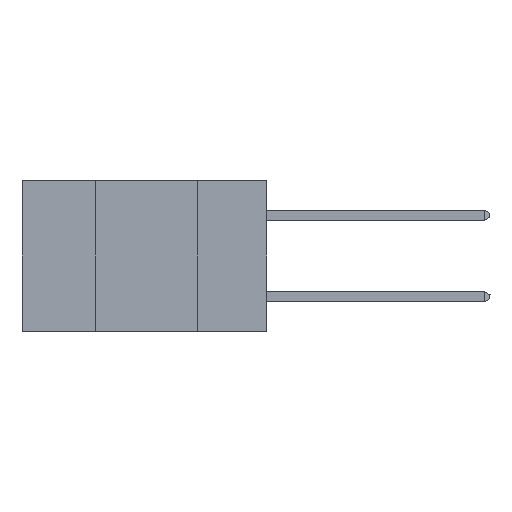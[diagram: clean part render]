
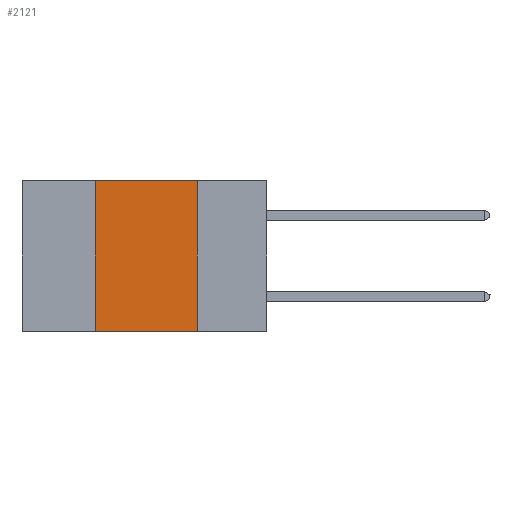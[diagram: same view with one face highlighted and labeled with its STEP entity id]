
A CAD part, left-side view. The second image highlights one B-rep face of the part: STEP entity #2121.
In plain terms, the highlighted planar face has unit normal (-1, 0, 0).
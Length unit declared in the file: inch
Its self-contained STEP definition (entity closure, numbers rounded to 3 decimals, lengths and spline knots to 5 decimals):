
#1467 = LINE ( 'NONE', #8343, #33028 ) ;
#2121 = ADVANCED_FACE ( 'NONE', ( #2876 ), #19632, .F. ) ;
#2876 = FACE_OUTER_BOUND ( 'NONE', #6727, .T. ) ;
#3193 = VECTOR ( 'NONE', #22017, 39.37008 ) ;
#6084 = LINE ( 'NONE', #10353, #6583 ) ;
#6583 = VECTOR ( 'NONE', #26523, 39.37008 ) ;
#6727 = EDGE_LOOP ( 'NONE', ( #13665, #14573, #33638, #40450 ) ) ;
#7032 = EDGE_CURVE ( 'NONE', #20802, #23685, #1467, .T. ) ;
#8343 = CARTESIAN_POINT ( 'NONE',  ( 0., 0.6, 0. ) ) ;
#10353 = CARTESIAN_POINT ( 'NONE',  ( 0., 0.42, 0. ) ) ;
#10369 = DIRECTION ( 'NONE',  ( 1., 0., 0. ) ) ;
#13665 = ORIENTED_EDGE ( 'NONE', *, *, #32735, .F. ) ;
#14012 = VERTEX_POINT ( 'NONE', #22303 ) ;
#14573 = ORIENTED_EDGE ( 'NONE', *, *, #7032, .F. ) ;
#19632 = PLANE ( 'NONE',  #36385 ) ;
#20323 = CARTESIAN_POINT ( 'NONE',  ( 0., 0.6, 0. ) ) ;
#20802 = VERTEX_POINT ( 'NONE', #41307 ) ;
#22017 = DIRECTION ( 'NONE',  ( 0., 0., -1. ) ) ;
#22303 = CARTESIAN_POINT ( 'NONE',  ( 0., 0.17, -0.37 ) ) ;
#22435 = CARTESIAN_POINT ( 'NONE',  ( 0., 0.17, 0. ) ) ;
#22905 = DIRECTION ( 'NONE',  ( 0., 0., -1. ) ) ;
#23334 = DIRECTION ( 'NONE',  ( 0., -1., 0. ) ) ;
#23685 = VERTEX_POINT ( 'NONE', #26655 ) ;
#24269 = DIRECTION ( 'NONE',  ( 0., -1., 0. ) ) ;
#26290 = CARTESIAN_POINT ( 'NONE',  ( 0., 0.6, -0.37 ) ) ;
#26523 = DIRECTION ( 'NONE',  ( 0., 0., 1. ) ) ;
#26655 = CARTESIAN_POINT ( 'NONE',  ( 0., 0.17, 0. ) ) ;
#26950 = EDGE_CURVE ( 'NONE', #27329, #14012, #39740, .T. ) ;
#27329 = VERTEX_POINT ( 'NONE', #41108 ) ;
#27575 = EDGE_CURVE ( 'NONE', #27329, #20802, #6084, .T. ) ;
#32603 = VECTOR ( 'NONE', #23334, 39.37008 ) ;
#32735 = EDGE_CURVE ( 'NONE', #23685, #14012, #34162, .T. ) ;
#33028 = VECTOR ( 'NONE', #24269, 39.37008 ) ;
#33638 = ORIENTED_EDGE ( 'NONE', *, *, #27575, .F. ) ;
#34162 = LINE ( 'NONE', #22435, #3193 ) ;
#36385 = AXIS2_PLACEMENT_3D ( 'NONE', #20323, #10369, #22905 ) ;
#39740 = LINE ( 'NONE', #26290, #32603 ) ;
#40450 = ORIENTED_EDGE ( 'NONE', *, *, #26950, .T. ) ;
#41108 = CARTESIAN_POINT ( 'NONE',  ( 0., 0.42, -0.37 ) ) ;
#41307 = CARTESIAN_POINT ( 'NONE',  ( 0., 0.42, 0. ) ) ;
